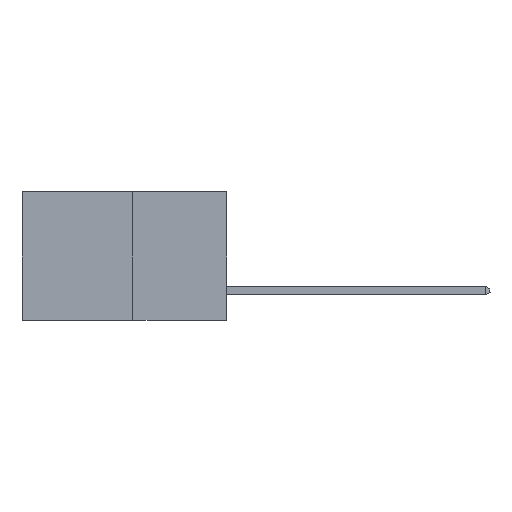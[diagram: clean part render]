
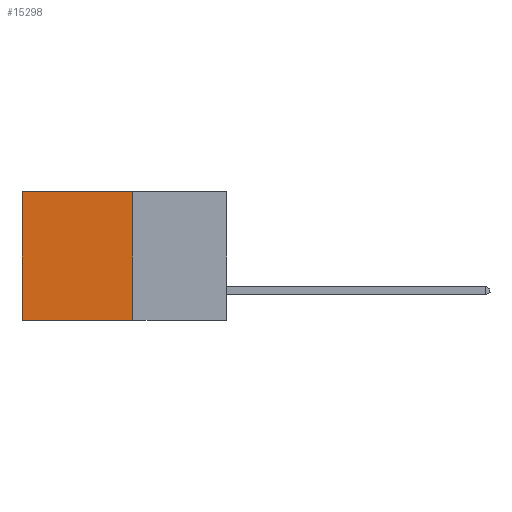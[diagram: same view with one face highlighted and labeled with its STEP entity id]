
A CAD part, left-side view. The second image highlights one B-rep face of the part: STEP entity #15298.
In plain terms, the highlighted planar face has unit normal (-1, 0, 0).
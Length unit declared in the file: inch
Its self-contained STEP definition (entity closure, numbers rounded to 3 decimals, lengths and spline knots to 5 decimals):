
#188 = PLANE ( 'NONE',  #2504 ) ;
#231 = EDGE_CURVE ( 'NONE', #6389, #4999, #1612, .T. ) ;
#1132 = CARTESIAN_POINT ( 'NONE',  ( 0.277, 0.27, 0. ) ) ;
#1253 = FACE_OUTER_BOUND ( 'NONE', #10717, .T. ) ;
#1406 = VERTEX_POINT ( 'NONE', #10725 ) ;
#1426 = DIRECTION ( 'NONE',  ( 1., 0., 0. ) ) ;
#1456 = CARTESIAN_POINT ( 'NONE',  ( 0.277, 0.27, -0.37 ) ) ;
#1612 = LINE ( 'NONE', #1456, #13888 ) ;
#2504 = AXIS2_PLACEMENT_3D ( 'NONE', #7448, #1426, #9842 ) ;
#3638 = ORIENTED_EDGE ( 'NONE', *, *, #6714, .T. ) ;
#3990 = CARTESIAN_POINT ( 'NONE',  ( 0.277, 0.59, -0.37 ) ) ;
#4036 = ORIENTED_EDGE ( 'NONE', *, *, #14391, .T. ) ;
#4301 = DIRECTION ( 'NONE',  ( 0., 0., -1. ) ) ;
#4371 = VECTOR ( 'NONE', #8796, 39.37008 ) ;
#4519 = CARTESIAN_POINT ( 'NONE',  ( 0.277, 0.59, -0.37 ) ) ;
#4746 = LINE ( 'NONE', #4996, #11070 ) ;
#4996 = CARTESIAN_POINT ( 'NONE',  ( 0.277, 0.27, -0.37 ) ) ;
#4999 = VERTEX_POINT ( 'NONE', #6724 ) ;
#6019 = EDGE_CURVE ( 'NONE', #4999, #8859, #4746, .T. ) ;
#6389 = VERTEX_POINT ( 'NONE', #6847 ) ;
#6714 = EDGE_CURVE ( 'NONE', #1406, #8859, #13779, .T. ) ;
#6724 = CARTESIAN_POINT ( 'NONE',  ( 0.277, 0.27, -0.37 ) ) ;
#6826 = ORIENTED_EDGE ( 'NONE', *, *, #6019, .F. ) ;
#6847 = CARTESIAN_POINT ( 'NONE',  ( 0.277, 0.27, 0. ) ) ;
#7081 = DIRECTION ( 'NONE',  ( 0., 1., 0. ) ) ;
#7448 = CARTESIAN_POINT ( 'NONE',  ( 0.277, 0.27, -0.37 ) ) ;
#8456 = LINE ( 'NONE', #1132, #12327 ) ;
#8796 = DIRECTION ( 'NONE',  ( 0., 0., -1. ) ) ;
#8859 = VERTEX_POINT ( 'NONE', #4519 ) ;
#9546 = DIRECTION ( 'NONE',  ( 0., 1., 0. ) ) ;
#9842 = DIRECTION ( 'NONE',  ( 0., 0., -1. ) ) ;
#10717 = EDGE_LOOP ( 'NONE', ( #3638, #6826, #13080, #4036 ) ) ;
#10725 = CARTESIAN_POINT ( 'NONE',  ( 0.277, 0.59, 0. ) ) ;
#11070 = VECTOR ( 'NONE', #7081, 39.37008 ) ;
#12327 = VECTOR ( 'NONE', #9546, 39.37008 ) ;
#13080 = ORIENTED_EDGE ( 'NONE', *, *, #231, .F. ) ;
#13779 = LINE ( 'NONE', #3990, #4371 ) ;
#13888 = VECTOR ( 'NONE', #4301, 39.37008 ) ;
#14391 = EDGE_CURVE ( 'NONE', #6389, #1406, #8456, .T. ) ;
#15298 = ADVANCED_FACE ( 'NONE', ( #1253 ), #188, .F. ) ;
